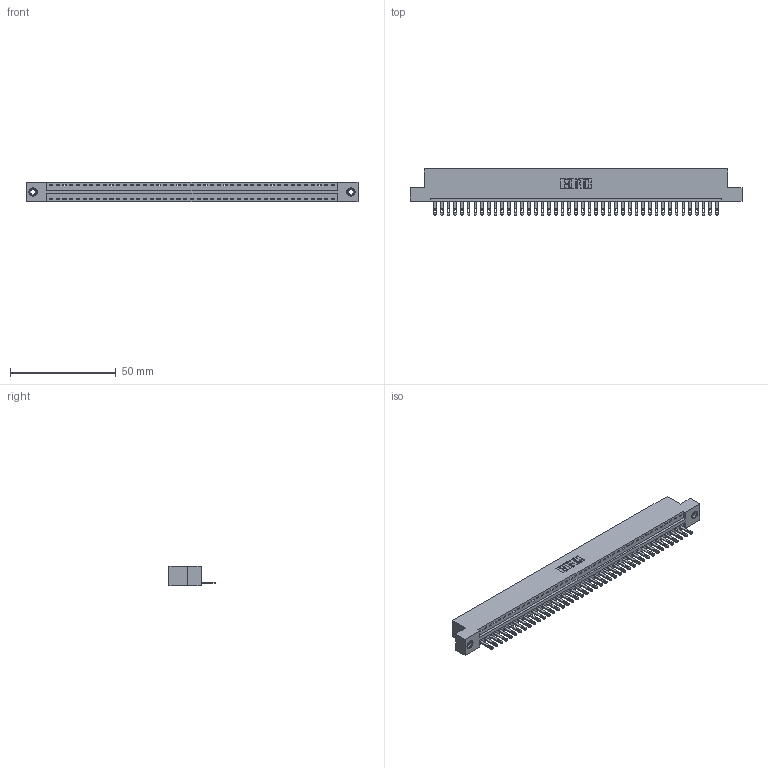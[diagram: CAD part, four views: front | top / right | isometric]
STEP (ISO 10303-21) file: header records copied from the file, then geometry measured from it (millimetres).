
FILE_DESCRIPTION (( 'STEP AP203' ), '1' );
FILE_NAME ('346-043-500-108.STEP', '2022-05-09T15:09:01', ( '' ), ( '' ), 'SwSTEP 2.0', 'SolidWorks 2020', '' );
FILE_SCHEMA (( 'CONFIG_CONTROL_DESIGN' ));
Length unit declared in the file: inch
Products named in the file (4): 345-250-001_345-250-003-102; 345-292-001_345-293-100; 346 Part_Flush Mounting Lugs - 0.156 Dia-TI; 346-043-500-108
Assembly tree (46 placements, depth 2):
  346-043-500-108
    346 Part_Flush Mounting Lugs - 0.156 Dia-TI
    345-292-001_345-293-100  x43
    345-250-001_345-250-003-102  x2
Bounding box: 157.1 x 21.84 x 9.4 mm (x, y, z)
Volume: 15064.8 mm3; surface area: 18961.9 mm2
Topology: 46 solids, 46 shells, 2504 faces, 7689 edges, 5118 vertices
Faces by surface type: plane 1570, cylinder 918, cone 12, torus 4
Entity records: 27668 total; most frequent: CARTESIAN_POINT 4724, ORIENTED_EDGE 4694, DIRECTION 4195, EDGE_CURVE 2347, VECTOR 2019, LINE 2019, VERTEX_POINT 1560, AXIS2_PLACEMENT_3D 1088
